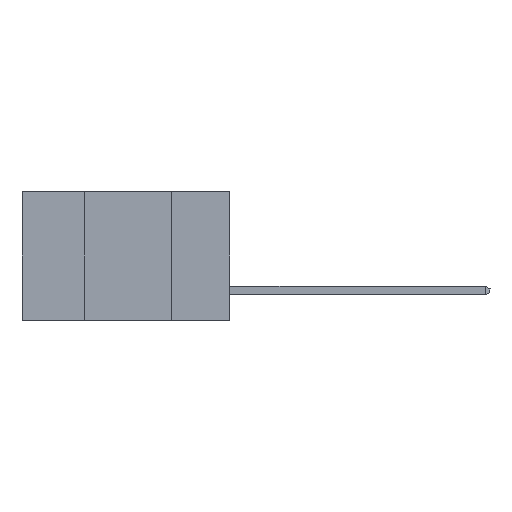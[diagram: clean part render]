
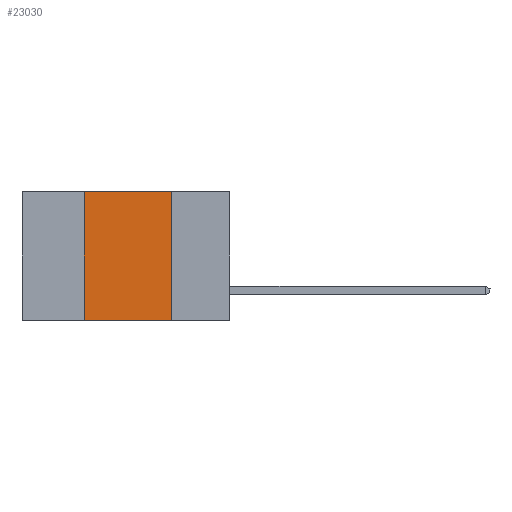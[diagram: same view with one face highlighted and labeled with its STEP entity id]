
A CAD part, left-side view. The second image highlights one B-rep face of the part: STEP entity #23030.
In plain terms, the highlighted planar face has unit normal (-1, 0, 0).
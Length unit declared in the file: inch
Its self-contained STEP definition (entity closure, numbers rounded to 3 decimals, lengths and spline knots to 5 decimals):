
#1574 = CARTESIAN_POINT ( 'NONE',  ( 0., 0.6, 0. ) ) ;
#2502 = EDGE_CURVE ( 'NONE', #8166, #8156, #15171, .T. ) ;
#3674 = AXIS2_PLACEMENT_3D ( 'NONE', #19350, #9537, #17601 ) ;
#4070 = CARTESIAN_POINT ( 'NONE',  ( 0., 0.42, -0.37 ) ) ;
#4195 = CARTESIAN_POINT ( 'NONE',  ( 0., 0.17, -0.37 ) ) ;
#4267 = ORIENTED_EDGE ( 'NONE', *, *, #2502, .T. ) ;
#4496 = EDGE_LOOP ( 'NONE', ( #9408, #16140, #18892, #4267 ) ) ;
#5133 = CARTESIAN_POINT ( 'NONE',  ( 0., 0.6, -0.37 ) ) ;
#5265 = VECTOR ( 'NONE', #14739, 39.37008 ) ;
#5642 = DIRECTION ( 'NONE',  ( 0., -1., 0. ) ) ;
#6770 = LINE ( 'NONE', #13104, #13832 ) ;
#6998 = VERTEX_POINT ( 'NONE', #10125 ) ;
#8156 = VERTEX_POINT ( 'NONE', #4195 ) ;
#8166 = VERTEX_POINT ( 'NONE', #4070 ) ;
#8622 = EDGE_CURVE ( 'NONE', #6998, #8156, #6770, .T. ) ;
#8891 = DIRECTION ( 'NONE',  ( 0., 0., -1. ) ) ;
#9251 = VERTEX_POINT ( 'NONE', #11714 ) ;
#9408 = ORIENTED_EDGE ( 'NONE', *, *, #8622, .F. ) ;
#9537 = DIRECTION ( 'NONE',  ( 1., 0., 0. ) ) ;
#10125 = CARTESIAN_POINT ( 'NONE',  ( 0., 0.17, 0. ) ) ;
#10675 = VECTOR ( 'NONE', #5642, 39.37008 ) ;
#11182 = CARTESIAN_POINT ( 'NONE',  ( 0., 0.42, -0.37 ) ) ;
#11714 = CARTESIAN_POINT ( 'NONE',  ( 0., 0.42, 0. ) ) ;
#13104 = CARTESIAN_POINT ( 'NONE',  ( 0., 0.17, -0.37 ) ) ;
#13181 = DIRECTION ( 'NONE',  ( 0., -1., 0. ) ) ;
#13696 = LINE ( 'NONE', #1574, #10675 ) ;
#13832 = VECTOR ( 'NONE', #8891, 39.37008 ) ;
#14739 = DIRECTION ( 'NONE',  ( 0., 0., 1. ) ) ;
#14871 = LINE ( 'NONE', #11182, #5265 ) ;
#15171 = LINE ( 'NONE', #5133, #16929 ) ;
#16140 = ORIENTED_EDGE ( 'NONE', *, *, #18611, .F. ) ;
#16929 = VECTOR ( 'NONE', #13181, 39.37008 ) ;
#17601 = DIRECTION ( 'NONE',  ( 0., 0., -1. ) ) ;
#18611 = EDGE_CURVE ( 'NONE', #9251, #6998, #13696, .T. ) ;
#18892 = ORIENTED_EDGE ( 'NONE', *, *, #20224, .F. ) ;
#19350 = CARTESIAN_POINT ( 'NONE',  ( 0., 0.6, 0. ) ) ;
#20224 = EDGE_CURVE ( 'NONE', #8166, #9251, #14871, .T. ) ;
#23030 = ADVANCED_FACE ( 'NONE', ( #23556 ), #23679, .F. ) ;
#23556 = FACE_OUTER_BOUND ( 'NONE', #4496, .T. ) ;
#23679 = PLANE ( 'NONE',  #3674 ) ;
